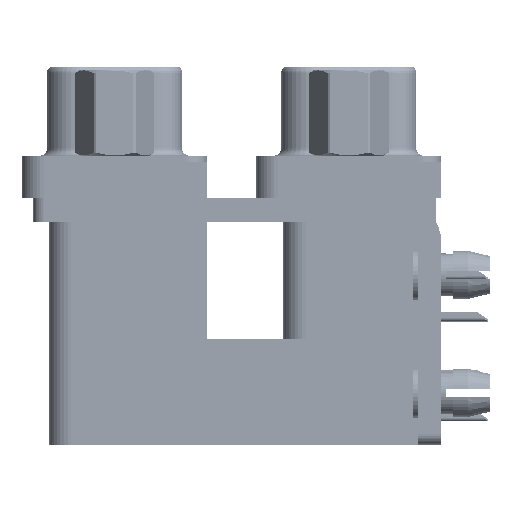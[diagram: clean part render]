
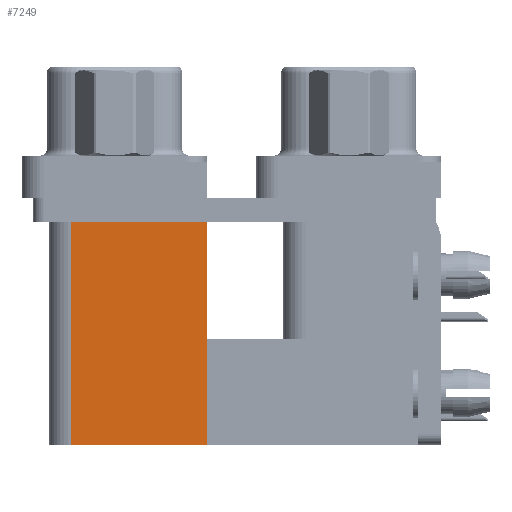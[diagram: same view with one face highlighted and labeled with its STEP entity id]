
A CAD part, left-side view. The second image highlights one B-rep face of the part: STEP entity #7249.
In plain terms, the highlighted planar face has unit normal (-1, 0, 0).
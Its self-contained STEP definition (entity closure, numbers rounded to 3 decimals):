
#3982 = CARTESIAN_POINT ( 'NONE',  ( 3.7, 18.8, -19.2 ) ) ;
#5426 = EDGE_CURVE ( 'NONE', #36613, #32747, #12185, .T. ) ;
#5674 = CARTESIAN_POINT ( 'NONE',  ( 3.7, 9.6, -19.2 ) ) ;
#7247 = CARTESIAN_POINT ( 'NONE',  ( 3.7, 18.8, -19.2 ) ) ;
#7249 = ADVANCED_FACE ( 'NONE', ( #42205 ), #38189, .F. ) ;
#10286 = ORIENTED_EDGE ( 'NONE', *, *, #43194, .F. ) ;
#12185 = LINE ( 'NONE', #41608, #25608 ) ;
#13547 = ORIENTED_EDGE ( 'NONE', *, *, #27003, .T. ) ;
#14187 = DIRECTION ( 'NONE',  ( 0., 1., 0. ) ) ;
#15626 = VERTEX_POINT ( 'NONE', #3982 ) ;
#15976 = EDGE_CURVE ( 'NONE', #15626, #38936, #43316, .T. ) ;
#16126 = CARTESIAN_POINT ( 'NONE',  ( 3.7, 9.6, -2.5 ) ) ;
#19624 = CARTESIAN_POINT ( 'NONE',  ( 3.7, 9.6, -2.5 ) ) ;
#21524 = LINE ( 'NONE', #36033, #42778 ) ;
#21691 = DIRECTION ( 'NONE',  ( 0., 0., 1. ) ) ;
#21808 = EDGE_LOOP ( 'NONE', ( #13547, #32419, #10286, #28342 ) ) ;
#24420 = LINE ( 'NONE', #16126, #25554 ) ;
#25554 = VECTOR ( 'NONE', #27281, 1000. ) ;
#25608 = VECTOR ( 'NONE', #29977, 1000. ) ;
#27003 = EDGE_CURVE ( 'NONE', #32747, #38936, #24420, .T. ) ;
#27281 = DIRECTION ( 'NONE',  ( 0., 1., 0. ) ) ;
#27732 = DIRECTION ( 'NONE',  ( 0., 0., -1. ) ) ;
#28342 = ORIENTED_EDGE ( 'NONE', *, *, #5426, .T. ) ;
#29977 = DIRECTION ( 'NONE',  ( 0., 0., 1. ) ) ;
#32419 = ORIENTED_EDGE ( 'NONE', *, *, #15976, .F. ) ;
#32747 = VERTEX_POINT ( 'NONE', #19624 ) ;
#33252 = CARTESIAN_POINT ( 'NONE',  ( 3.7, 9.6, -19.2 ) ) ;
#34436 = VECTOR ( 'NONE', #21691, 1000. ) ;
#34631 = DIRECTION ( 'NONE',  ( 1., 0., 0. ) ) ;
#35492 = AXIS2_PLACEMENT_3D ( 'NONE', #5674, #34631, #27732 ) ;
#36033 = CARTESIAN_POINT ( 'NONE',  ( 3.7, 9.6, -19.2 ) ) ;
#36613 = VERTEX_POINT ( 'NONE', #33252 ) ;
#38189 = PLANE ( 'NONE',  #35492 ) ;
#38936 = VERTEX_POINT ( 'NONE', #46931 ) ;
#41608 = CARTESIAN_POINT ( 'NONE',  ( 3.7, 9.6, -19.2 ) ) ;
#42205 = FACE_OUTER_BOUND ( 'NONE', #21808, .T. ) ;
#42778 = VECTOR ( 'NONE', #14187, 1000. ) ;
#43194 = EDGE_CURVE ( 'NONE', #36613, #15626, #21524, .T. ) ;
#43316 = LINE ( 'NONE', #7247, #34436 ) ;
#46931 = CARTESIAN_POINT ( 'NONE',  ( 3.7, 18.8, -2.5 ) ) ;
